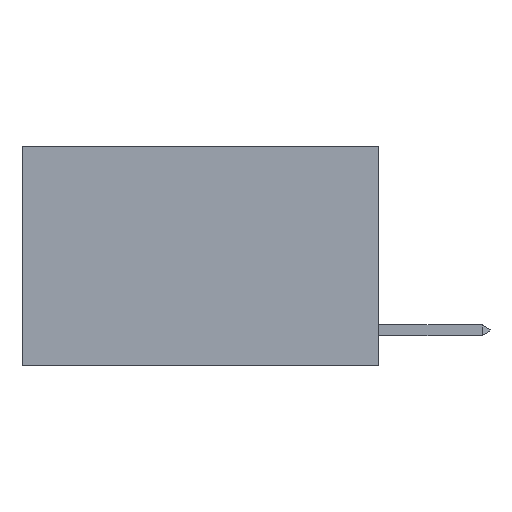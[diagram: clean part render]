
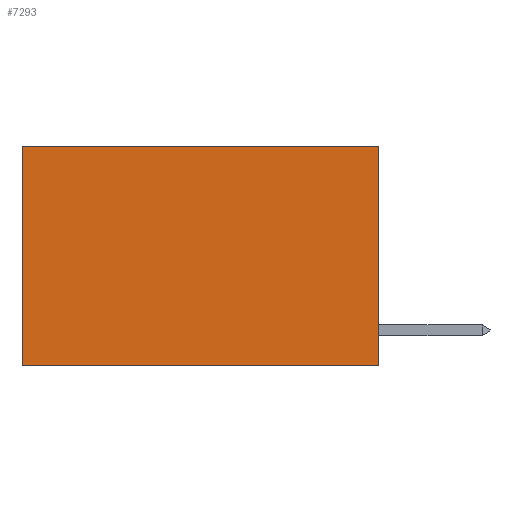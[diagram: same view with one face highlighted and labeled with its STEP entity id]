
A CAD part, left-side view. The second image highlights one B-rep face of the part: STEP entity #7293.
In plain terms, the highlighted planar face has unit normal (-1, 0, 0).
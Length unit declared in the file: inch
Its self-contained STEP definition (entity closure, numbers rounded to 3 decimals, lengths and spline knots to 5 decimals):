
#1110 = LINE ( 'NONE', #13756, #16512 ) ;
#1277 = CARTESIAN_POINT ( 'NONE',  ( 0.2625, 0.6, 0. ) ) ;
#1838 = EDGE_CURVE ( 'NONE', #2799, #15685, #13648, .T. ) ;
#2799 = VERTEX_POINT ( 'NONE', #12026 ) ;
#3079 = EDGE_CURVE ( 'NONE', #4596, #2799, #12892, .T. ) ;
#3139 = CARTESIAN_POINT ( 'NONE',  ( 0.2625, 0., 0. ) ) ;
#3938 = CARTESIAN_POINT ( 'NONE',  ( 0.2625, 0., 0. ) ) ;
#4596 = VERTEX_POINT ( 'NONE', #3139 ) ;
#4934 = DIRECTION ( 'NONE',  ( 0., 0., -1. ) ) ;
#5314 = CARTESIAN_POINT ( 'NONE',  ( 0.2625, 0.6, -0.37 ) ) ;
#6428 = DIRECTION ( 'NONE',  ( 0., 0., -1. ) ) ;
#7293 = ADVANCED_FACE ( 'NONE', ( #16978 ), #19874, .F. ) ;
#7489 = CARTESIAN_POINT ( 'NONE',  ( 0.2625, 0., -0.37 ) ) ;
#10627 = ORIENTED_EDGE ( 'NONE', *, *, #20435, .T. ) ;
#10952 = VERTEX_POINT ( 'NONE', #1277 ) ;
#11426 = VECTOR ( 'NONE', #6428, 39.37008 ) ;
#11984 = DIRECTION ( 'NONE',  ( 0., 0., -1. ) ) ;
#12026 = CARTESIAN_POINT ( 'NONE',  ( 0.2625, 0., -0.37 ) ) ;
#12433 = DIRECTION ( 'NONE',  ( 0., 1., 0. ) ) ;
#12448 = VECTOR ( 'NONE', #12433, 39.37008 ) ;
#12892 = LINE ( 'NONE', #14249, #11426 ) ;
#13633 = ORIENTED_EDGE ( 'NONE', *, *, #1838, .F. ) ;
#13648 = LINE ( 'NONE', #7489, #12448 ) ;
#13756 = CARTESIAN_POINT ( 'NONE',  ( 0.2625, 0., 0. ) ) ;
#14249 = CARTESIAN_POINT ( 'NONE',  ( 0.2625, 0., 0. ) ) ;
#14428 = ORIENTED_EDGE ( 'NONE', *, *, #3079, .F. ) ;
#14484 = EDGE_LOOP ( 'NONE', ( #15196, #13633, #14428, #10627 ) ) ;
#15064 = DIRECTION ( 'NONE',  ( 1., 0., 0. ) ) ;
#15196 = ORIENTED_EDGE ( 'NONE', *, *, #19465, .T. ) ;
#15311 = LINE ( 'NONE', #17497, #17278 ) ;
#15685 = VERTEX_POINT ( 'NONE', #5314 ) ;
#16512 = VECTOR ( 'NONE', #16986, 39.37008 ) ;
#16978 = FACE_OUTER_BOUND ( 'NONE', #14484, .T. ) ;
#16986 = DIRECTION ( 'NONE',  ( 0., 1., 0. ) ) ;
#17278 = VECTOR ( 'NONE', #4934, 39.37008 ) ;
#17497 = CARTESIAN_POINT ( 'NONE',  ( 0.2625, 0.6, 0. ) ) ;
#19059 = AXIS2_PLACEMENT_3D ( 'NONE', #3938, #15064, #11984 ) ;
#19465 = EDGE_CURVE ( 'NONE', #10952, #15685, #15311, .T. ) ;
#19874 = PLANE ( 'NONE',  #19059 ) ;
#20435 = EDGE_CURVE ( 'NONE', #4596, #10952, #1110, .T. ) ;
